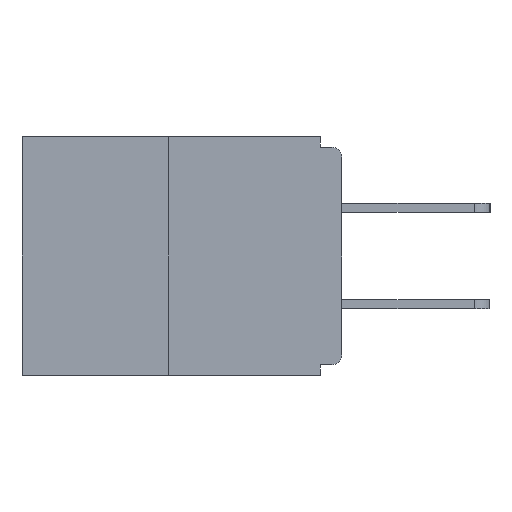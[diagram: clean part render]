
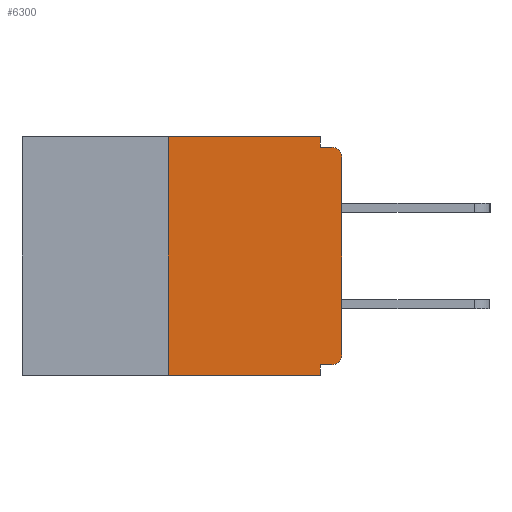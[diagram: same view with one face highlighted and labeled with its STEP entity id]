
A CAD part, left-side view. The second image highlights one B-rep face of the part: STEP entity #6300.
In plain terms, the highlighted planar face has unit normal (-1, 0, 0).
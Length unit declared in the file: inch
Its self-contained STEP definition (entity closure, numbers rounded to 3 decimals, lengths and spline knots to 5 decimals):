
#43 = CARTESIAN_POINT ( 'NONE',  ( 0., 0.25, -0.343 ) ) ;
#51 = VERTEX_POINT ( 'NONE', #20790 ) ;
#1162 = DIRECTION ( 'NONE',  ( 0., 0., 1. ) ) ;
#1412 = EDGE_CURVE ( 'NONE', #27246, #12047, #19444, .T. ) ;
#1442 = VERTEX_POINT ( 'NONE', #8575 ) ;
#1612 = AXIS2_PLACEMENT_3D ( 'NONE', #24377, #20129, #28895 ) ;
#1672 = DIRECTION ( 'NONE',  ( -1., 0., 0. ) ) ;
#2389 = LINE ( 'NONE', #23321, #17240 ) ;
#2595 = ORIENTED_EDGE ( 'NONE', *, *, #20434, .T. ) ;
#2987 = EDGE_CURVE ( 'NONE', #14288, #18608, #2389, .T. ) ;
#3189 = DIRECTION ( 'NONE',  ( 0., 1., 0. ) ) ;
#3929 = DIRECTION ( 'NONE',  ( 0., 0., -1. ) ) ;
#4592 = VECTOR ( 'NONE', #24167, 39.37008 ) ;
#4857 = VERTEX_POINT ( 'NONE', #43 ) ;
#5323 = VECTOR ( 'NONE', #3929, 39.37008 ) ;
#5426 = ORIENTED_EDGE ( 'NONE', *, *, #6148, .F. ) ;
#5518 = CIRCLE ( 'NONE', #1612, 0.015 ) ;
#6082 = CARTESIAN_POINT ( 'NONE',  ( 0., 0.46, 0. ) ) ;
#6148 = EDGE_CURVE ( 'NONE', #1442, #20152, #20899, .T. ) ;
#6300 = ADVANCED_FACE ( 'NONE', ( #17003 ), #25008, .F. ) ;
#6759 = EDGE_CURVE ( 'NONE', #4857, #51, #18738, .T. ) ;
#7475 = CARTESIAN_POINT ( 'NONE',  ( 0., 0.46, -0.343 ) ) ;
#8020 = CARTESIAN_POINT ( 'NONE',  ( 0., 0.25, 0. ) ) ;
#8300 = AXIS2_PLACEMENT_3D ( 'NONE', #9491, #18576, #11472 ) ;
#8575 = CARTESIAN_POINT ( 'NONE',  ( 0., 0.031, -0.015 ) ) ;
#8829 = CARTESIAN_POINT ( 'NONE',  ( 0., 0.031, -0.343 ) ) ;
#9198 = EDGE_LOOP ( 'NONE', ( #28144, #13928, #19012, #24937, #29152, #2595, #20239, #20985, #5426, #21162 ) ) ;
#9491 = CARTESIAN_POINT ( 'NONE',  ( 0., 0.46, 0. ) ) ;
#11449 = VERTEX_POINT ( 'NONE', #8020 ) ;
#11472 = DIRECTION ( 'NONE',  ( 0., 0., -1. ) ) ;
#12047 = VERTEX_POINT ( 'NONE', #20257 ) ;
#12412 = EDGE_CURVE ( 'NONE', #20274, #1442, #17339, .T. ) ;
#12444 = DIRECTION ( 'NONE',  ( 0., 0., 1. ) ) ;
#12620 = AXIS2_PLACEMENT_3D ( 'NONE', #15091, #1672, #28499 ) ;
#13138 = VECTOR ( 'NONE', #12444, 39.37008 ) ;
#13273 = DIRECTION ( 'NONE',  ( 0., -1., 0. ) ) ;
#13928 = ORIENTED_EDGE ( 'NONE', *, *, #26233, .F. ) ;
#14288 = VERTEX_POINT ( 'NONE', #19179 ) ;
#14696 = CARTESIAN_POINT ( 'NONE',  ( 0., 0., 0. ) ) ;
#14915 = CARTESIAN_POINT ( 'NONE',  ( 0., 0.25, 0. ) ) ;
#15091 = CARTESIAN_POINT ( 'NONE',  ( 0., 0.015, -0.03 ) ) ;
#15545 = EDGE_CURVE ( 'NONE', #18608, #51, #18908, .T. ) ;
#16124 = CARTESIAN_POINT ( 'NONE',  ( 0., 0., -0.313 ) ) ;
#17003 = FACE_OUTER_BOUND ( 'NONE', #9198, .T. ) ;
#17240 = VECTOR ( 'NONE', #3189, 39.37008 ) ;
#17339 = LINE ( 'NONE', #17464, #5323 ) ;
#17464 = CARTESIAN_POINT ( 'NONE',  ( 0., 0.031, 0. ) ) ;
#18036 = VECTOR ( 'NONE', #18543, 39.37008 ) ;
#18543 = DIRECTION ( 'NONE',  ( 0., -1., 0. ) ) ;
#18576 = DIRECTION ( 'NONE',  ( 1., 0., 0. ) ) ;
#18608 = VERTEX_POINT ( 'NONE', #19573 ) ;
#18738 = LINE ( 'NONE', #7475, #18036 ) ;
#18908 = LINE ( 'NONE', #8829, #27374 ) ;
#19012 = ORIENTED_EDGE ( 'NONE', *, *, #6759, .T. ) ;
#19179 = CARTESIAN_POINT ( 'NONE',  ( 0., 0.015, -0.328 ) ) ;
#19444 = LINE ( 'NONE', #14696, #27574 ) ;
#19573 = CARTESIAN_POINT ( 'NONE',  ( 0., 0.031, -0.328 ) ) ;
#19838 = CARTESIAN_POINT ( 'NONE',  ( 0., 0.031, 0. ) ) ;
#20129 = DIRECTION ( 'NONE',  ( -1., 0., 0. ) ) ;
#20152 = VERTEX_POINT ( 'NONE', #28313 ) ;
#20239 = ORIENTED_EDGE ( 'NONE', *, *, #1412, .T. ) ;
#20257 = CARTESIAN_POINT ( 'NONE',  ( 0., 0., -0.03 ) ) ;
#20274 = VERTEX_POINT ( 'NONE', #19838 ) ;
#20280 = DIRECTION ( 'NONE',  ( 0., 0., -1. ) ) ;
#20434 = EDGE_CURVE ( 'NONE', #14288, #27246, #5518, .T. ) ;
#20790 = CARTESIAN_POINT ( 'NONE',  ( 0., 0.031, -0.343 ) ) ;
#20899 = LINE ( 'NONE', #22539, #26202 ) ;
#20985 = ORIENTED_EDGE ( 'NONE', *, *, #23163, .T. ) ;
#21162 = ORIENTED_EDGE ( 'NONE', *, *, #12412, .F. ) ;
#22539 = CARTESIAN_POINT ( 'NONE',  ( 0., 0., -0.015 ) ) ;
#23163 = EDGE_CURVE ( 'NONE', #12047, #20152, #28671, .T. ) ;
#23321 = CARTESIAN_POINT ( 'NONE',  ( 0., 0., -0.328 ) ) ;
#24167 = DIRECTION ( 'NONE',  ( 0., -1., 0. ) ) ;
#24377 = CARTESIAN_POINT ( 'NONE',  ( 0., 0.015, -0.313 ) ) ;
#24937 = ORIENTED_EDGE ( 'NONE', *, *, #15545, .F. ) ;
#25008 = PLANE ( 'NONE',  #8300 ) ;
#26202 = VECTOR ( 'NONE', #13273, 39.37008 ) ;
#26233 = EDGE_CURVE ( 'NONE', #4857, #11449, #28294, .T. ) ;
#26963 = EDGE_CURVE ( 'NONE', #11449, #20274, #27207, .T. ) ;
#27207 = LINE ( 'NONE', #6082, #4592 ) ;
#27246 = VERTEX_POINT ( 'NONE', #16124 ) ;
#27374 = VECTOR ( 'NONE', #20280, 39.37008 ) ;
#27574 = VECTOR ( 'NONE', #1162, 39.37008 ) ;
#28144 = ORIENTED_EDGE ( 'NONE', *, *, #26963, .F. ) ;
#28294 = LINE ( 'NONE', #14915, #13138 ) ;
#28313 = CARTESIAN_POINT ( 'NONE',  ( 0., 0.015, -0.015 ) ) ;
#28499 = DIRECTION ( 'NONE',  ( 0., 0., -1. ) ) ;
#28671 = CIRCLE ( 'NONE', #12620, 0.015 ) ;
#28895 = DIRECTION ( 'NONE',  ( 0., 0., -1. ) ) ;
#29152 = ORIENTED_EDGE ( 'NONE', *, *, #2987, .F. ) ;
